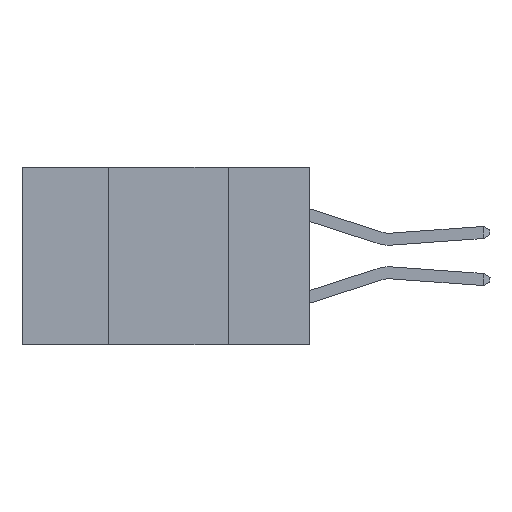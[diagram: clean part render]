
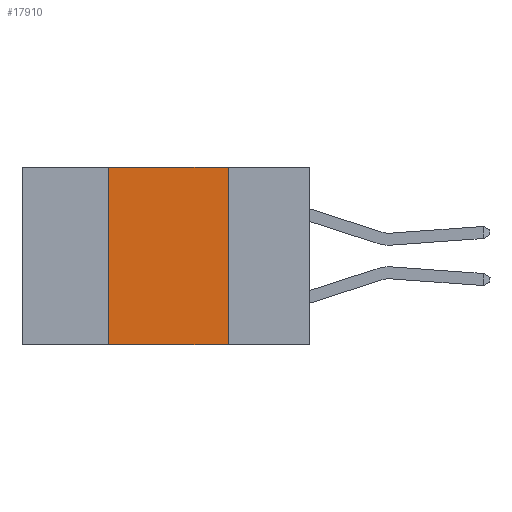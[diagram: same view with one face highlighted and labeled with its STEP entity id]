
A CAD part, left-side view. The second image highlights one B-rep face of the part: STEP entity #17910.
In plain terms, the highlighted planar face has unit normal (-1, 0, 0).
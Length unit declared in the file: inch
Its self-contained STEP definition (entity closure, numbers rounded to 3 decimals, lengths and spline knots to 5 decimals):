
#85 = EDGE_CURVE ( 'NONE', #3978, #14431, #5609, .T. ) ;
#311 = LINE ( 'NONE', #8672, #15558 ) ;
#437 = DIRECTION ( 'NONE',  ( 1., 0., 0. ) ) ;
#548 = ORIENTED_EDGE ( 'NONE', *, *, #13438, .T. ) ;
#561 = LINE ( 'NONE', #14257, #3095 ) ;
#674 = DIRECTION ( 'NONE',  ( 0., 0., -1. ) ) ;
#860 = CARTESIAN_POINT ( 'NONE',  ( 0., 0.42, 0. ) ) ;
#882 = CARTESIAN_POINT ( 'NONE',  ( 0., 0.6, 0. ) ) ;
#2231 = CARTESIAN_POINT ( 'NONE',  ( 0., 0.17, 0. ) ) ;
#2385 = EDGE_CURVE ( 'NONE', #2783, #3978, #561, .T. ) ;
#2783 = VERTEX_POINT ( 'NONE', #860 ) ;
#3095 = VECTOR ( 'NONE', #11235, 39.37008 ) ;
#3809 = ORIENTED_EDGE ( 'NONE', *, *, #2385, .F. ) ;
#3978 = VERTEX_POINT ( 'NONE', #16936 ) ;
#4504 = FACE_OUTER_BOUND ( 'NONE', #11763, .T. ) ;
#5014 = VECTOR ( 'NONE', #9448, 39.37008 ) ;
#5609 = LINE ( 'NONE', #2231, #12983 ) ;
#6112 = CARTESIAN_POINT ( 'NONE',  ( 0., 0.42, -0.37 ) ) ;
#6646 = PLANE ( 'NONE',  #8860 ) ;
#8321 = DIRECTION ( 'NONE',  ( 0., 0., -1. ) ) ;
#8672 = CARTESIAN_POINT ( 'NONE',  ( 0., 0.42, 0. ) ) ;
#8860 = AXIS2_PLACEMENT_3D ( 'NONE', #882, #437, #8321 ) ;
#9448 = DIRECTION ( 'NONE',  ( 0., -1., 0. ) ) ;
#11235 = DIRECTION ( 'NONE',  ( 0., -1., 0. ) ) ;
#11763 = EDGE_LOOP ( 'NONE', ( #13197, #3809, #16747, #548 ) ) ;
#12209 = CARTESIAN_POINT ( 'NONE',  ( 0., 0.6, -0.37 ) ) ;
#12983 = VECTOR ( 'NONE', #674, 39.37008 ) ;
#13095 = DIRECTION ( 'NONE',  ( 0., 0., 1. ) ) ;
#13197 = ORIENTED_EDGE ( 'NONE', *, *, #85, .F. ) ;
#13290 = VERTEX_POINT ( 'NONE', #6112 ) ;
#13438 = EDGE_CURVE ( 'NONE', #13290, #14431, #13768, .T. ) ;
#13768 = LINE ( 'NONE', #12209, #5014 ) ;
#14257 = CARTESIAN_POINT ( 'NONE',  ( 0., 0.6, 0. ) ) ;
#14431 = VERTEX_POINT ( 'NONE', #19076 ) ;
#15558 = VECTOR ( 'NONE', #13095, 39.37008 ) ;
#16747 = ORIENTED_EDGE ( 'NONE', *, *, #18807, .F. ) ;
#16936 = CARTESIAN_POINT ( 'NONE',  ( 0., 0.17, 0. ) ) ;
#17910 = ADVANCED_FACE ( 'NONE', ( #4504 ), #6646, .F. ) ;
#18807 = EDGE_CURVE ( 'NONE', #13290, #2783, #311, .T. ) ;
#19076 = CARTESIAN_POINT ( 'NONE',  ( 0., 0.17, -0.37 ) ) ;
